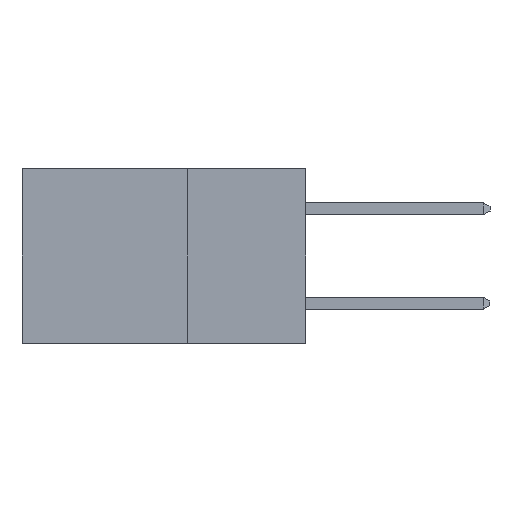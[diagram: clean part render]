
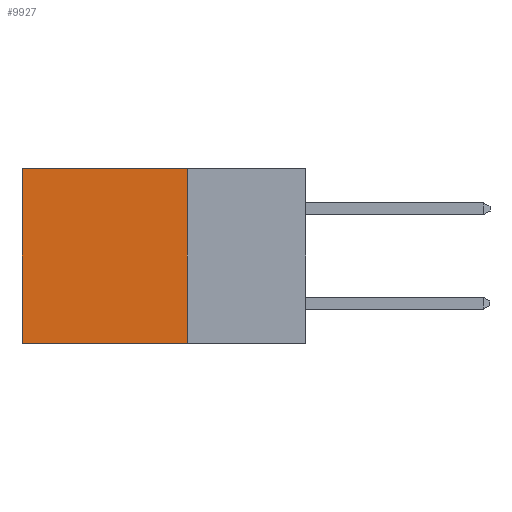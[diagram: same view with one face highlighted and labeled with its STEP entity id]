
A CAD part, left-side view. The second image highlights one B-rep face of the part: STEP entity #9927.
In plain terms, the highlighted planar face has unit normal (-1, 0, 0).
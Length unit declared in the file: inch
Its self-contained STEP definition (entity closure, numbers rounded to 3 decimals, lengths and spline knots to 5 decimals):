
#121 = CARTESIAN_POINT ( 'NONE',  ( 0.298, 0.25, 0. ) ) ;
#189 = DIRECTION ( 'NONE',  ( 0., 0., -1. ) ) ;
#1267 = DIRECTION ( 'NONE',  ( 1., 0., 0. ) ) ;
#1475 = VERTEX_POINT ( 'NONE', #5074 ) ;
#1489 = EDGE_CURVE ( 'NONE', #7745, #1475, #12800, .T. ) ;
#1880 = EDGE_CURVE ( 'NONE', #7745, #4636, #8118, .T. ) ;
#4354 = CARTESIAN_POINT ( 'NONE',  ( 0.298, 0.6, -0.37 ) ) ;
#4622 = CARTESIAN_POINT ( 'NONE',  ( 0.298, 0.25, 0. ) ) ;
#4636 = VERTEX_POINT ( 'NONE', #12660 ) ;
#4819 = ORIENTED_EDGE ( 'NONE', *, *, #1880, .F. ) ;
#5060 = VECTOR ( 'NONE', #14850, 39.37008 ) ;
#5074 = CARTESIAN_POINT ( 'NONE',  ( 0.298, 0.6, 0. ) ) ;
#5209 = CARTESIAN_POINT ( 'NONE',  ( 0.298, 0.25, 0. ) ) ;
#5226 = AXIS2_PLACEMENT_3D ( 'NONE', #121, #1267, #9558 ) ;
#6253 = ORIENTED_EDGE ( 'NONE', *, *, #14375, .T. ) ;
#7170 = PLANE ( 'NONE',  #5226 ) ;
#7745 = VERTEX_POINT ( 'NONE', #11720 ) ;
#7873 = ORIENTED_EDGE ( 'NONE', *, *, #8345, .F. ) ;
#8015 = CARTESIAN_POINT ( 'NONE',  ( 0.298, 0.25, -0.37 ) ) ;
#8118 = LINE ( 'NONE', #5209, #10818 ) ;
#8220 = FACE_OUTER_BOUND ( 'NONE', #11159, .T. ) ;
#8345 = EDGE_CURVE ( 'NONE', #4636, #12414, #14380, .T. ) ;
#8469 = LINE ( 'NONE', #13210, #11512 ) ;
#9558 = DIRECTION ( 'NONE',  ( 0., 0., -1. ) ) ;
#9779 = VECTOR ( 'NONE', #10284, 39.37008 ) ;
#9927 = ADVANCED_FACE ( 'NONE', ( #8220 ), #7170, .F. ) ;
#10284 = DIRECTION ( 'NONE',  ( 0., 1., 0. ) ) ;
#10818 = VECTOR ( 'NONE', #189, 39.37008 ) ;
#11159 = EDGE_LOOP ( 'NONE', ( #6253, #7873, #4819, #12521 ) ) ;
#11512 = VECTOR ( 'NONE', #14409, 39.37008 ) ;
#11720 = CARTESIAN_POINT ( 'NONE',  ( 0.298, 0.25, 0. ) ) ;
#12414 = VERTEX_POINT ( 'NONE', #4354 ) ;
#12521 = ORIENTED_EDGE ( 'NONE', *, *, #1489, .T. ) ;
#12660 = CARTESIAN_POINT ( 'NONE',  ( 0.298, 0.25, -0.37 ) ) ;
#12800 = LINE ( 'NONE', #4622, #9779 ) ;
#13210 = CARTESIAN_POINT ( 'NONE',  ( 0.298, 0.6, 0. ) ) ;
#14375 = EDGE_CURVE ( 'NONE', #1475, #12414, #8469, .T. ) ;
#14380 = LINE ( 'NONE', #8015, #5060 ) ;
#14409 = DIRECTION ( 'NONE',  ( 0., 0., -1. ) ) ;
#14850 = DIRECTION ( 'NONE',  ( 0., 1., 0. ) ) ;
